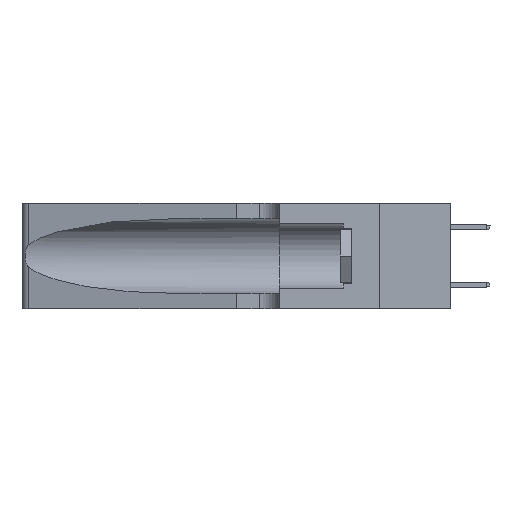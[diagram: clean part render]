
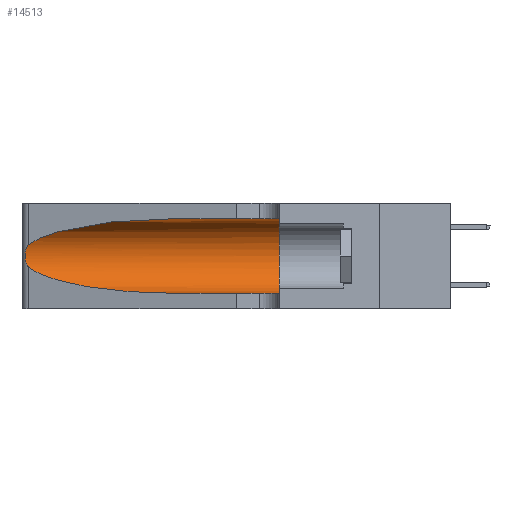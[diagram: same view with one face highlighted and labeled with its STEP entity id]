
A CAD part, left-side view. The second image highlights one B-rep face of the part: STEP entity #14513.
In plain terms, the highlighted cylindrical face has radius 3.308 mm (diameter 6.617 mm), a partial arc.
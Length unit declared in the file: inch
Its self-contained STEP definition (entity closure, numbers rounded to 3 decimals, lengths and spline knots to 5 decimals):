
#110 = DIRECTION ( 'NONE',  ( 0., -1., 0. ) ) ;
#166 = CIRCLE ( 'NONE', #18232, 0.13025 ) ;
#300 = LINE ( 'NONE', #17648, #17680 ) ;
#466 = EDGE_CURVE ( 'NONE', #22227, #18859, #23369, .T. ) ;
#804 = CARTESIAN_POINT ( 'NONE',  ( 0.25639, 1.23184, 0.21858 ) ) ;
#888 = ORIENTED_EDGE ( 'NONE', *, *, #16336, .F. ) ;
#924 = DIRECTION ( 'NONE',  ( 0., 0., -1. ) ) ;
#2369 = ORIENTED_EDGE ( 'NONE', *, *, #466, .T. ) ;
#2745 = VECTOR ( 'NONE', #110, 39.37008 ) ;
#2759 = VERTEX_POINT ( 'NONE', #21472 ) ;
#2931 = CARTESIAN_POINT ( 'NONE',  ( 0.26075, 1.23896, 0.178 ) ) ;
#5350 = VERTEX_POINT ( 'NONE', #18306 ) ;
#6581 = CARTESIAN_POINT ( 'NONE',  ( 0.25487, 1.22718, 0.14631 ) ) ;
#6843 = CYLINDRICAL_SURFACE ( 'NONE', #21247, 0.13025 ) ;
#7095 = CARTESIAN_POINT ( 'NONE',  ( 0.1305, 0.72297, 0.05475 ) ) ;
#8131 =( BOUNDED_CURVE ( )  B_SPLINE_CURVE ( 3, ( #22551, #12999, #22797, #11253 ),
 .UNSPECIFIED., .F., .F. ) 
 B_SPLINE_CURVE_WITH_KNOTS ( ( 4, 4 ),
 ( 1.5708, 2.84003 ),
 .UNSPECIFIED. ) 
 CURVE ( )  GEOMETRIC_REPRESENTATION_ITEM ( )  RATIONAL_B_SPLINE_CURVE ( ( 1., 0.87, 0.87, 1. ) ) 
 REPRESENTATION_ITEM ( '' )  );
#8192 = EDGE_LOOP ( 'NONE', ( #17746, #2369, #16391, #24027, #888, #19380 ) ) ;
#8236 = CARTESIAN_POINT ( 'NONE',  ( 0.25487, 1.22718, 0.22369 ) ) ;
#8818 = LINE ( 'NONE', #20715, #2745 ) ;
#8827 = CARTESIAN_POINT ( 'NONE',  ( 0.1305, 0.35, 0.185 ) ) ;
#10013 = CARTESIAN_POINT ( 'NONE',  ( 0.1305, 0.72297, 0.05475 ) ) ;
#10617 = CARTESIAN_POINT ( 'NONE',  ( 0.25487, 1.22718, 0.14631 ) ) ;
#10683 =( BOUNDED_CURVE ( )  B_SPLINE_CURVE ( 3, ( #10617, #10859, #10736, #7095 ),
 .UNSPECIFIED., .F., .T. ) 
 B_SPLINE_CURVE_WITH_KNOTS ( ( 4, 4 ),
 ( 3.44316, 4.71239 ),
 .UNSPECIFIED. ) 
 CURVE ( )  GEOMETRIC_REPRESENTATION_ITEM ( )  RATIONAL_B_SPLINE_CURVE ( ( 1., 0.87, 0.87, 1. ) ) 
 REPRESENTATION_ITEM ( '' )  );
#10736 = CARTESIAN_POINT ( 'NONE',  ( 0.18966, 0.96281, 0.05475 ) ) ;
#10859 = CARTESIAN_POINT ( 'NONE',  ( 0.2373, 1.15595, 0.08982 ) ) ;
#11253 = CARTESIAN_POINT ( 'NONE',  ( 0.25487, 1.22718, 0.22369 ) ) ;
#11676 = CARTESIAN_POINT ( 'NONE',  ( 0.25487, 1.22718, 0.14631 ) ) ;
#12350 = CARTESIAN_POINT ( 'NONE',  ( 0.1305, 0.72297, 0.31525 ) ) ;
#12591 = DIRECTION ( 'NONE',  ( 0., -1., 0. ) ) ;
#12599 = VERTEX_POINT ( 'NONE', #10013 ) ;
#12999 = CARTESIAN_POINT ( 'NONE',  ( 0.18966, 0.96281, 0.31525 ) ) ;
#13373 = EDGE_CURVE ( 'NONE', #12599, #2759, #8818, .T. ) ;
#13858 = CARTESIAN_POINT ( 'NONE',  ( 0.25787, 1.23484, 0.2124 ) ) ;
#14202 = DIRECTION ( 'NONE',  ( 0., 0., 1. ) ) ;
#14463 = CARTESIAN_POINT ( 'NONE',  ( 0.25487, 1.22718, 0.22369 ) ) ;
#14513 = ADVANCED_FACE ( 'NONE', ( #21786 ), #6843, .F. ) ;
#15771 = EDGE_CURVE ( 'NONE', #18040, #5350, #300, .T. ) ;
#15882 = CARTESIAN_POINT ( 'NONE',  ( 0.26017, 1.23833, 0.17102 ) ) ;
#16336 = EDGE_CURVE ( 'NONE', #5350, #2759, #166, .T. ) ;
#16391 = ORIENTED_EDGE ( 'NONE', *, *, #23026, .T. ) ;
#17648 = CARTESIAN_POINT ( 'NONE',  ( 0.1305, 1.61858, 0.31525 ) ) ;
#17680 = VECTOR ( 'NONE', #21291, 39.37008 ) ;
#17746 = ORIENTED_EDGE ( 'NONE', *, *, #22714, .T. ) ;
#18040 = VERTEX_POINT ( 'NONE', #12350 ) ;
#18232 = AXIS2_PLACEMENT_3D ( 'NONE', #8827, #23772, #14202 ) ;
#18265 = CARTESIAN_POINT ( 'NONE',  ( 0.1305, 1.61858, 0.185 ) ) ;
#18306 = CARTESIAN_POINT ( 'NONE',  ( 0.1305, 0.35, 0.31525 ) ) ;
#18859 = VERTEX_POINT ( 'NONE', #11676 ) ;
#19380 = ORIENTED_EDGE ( 'NONE', *, *, #15771, .F. ) ;
#19653 = CARTESIAN_POINT ( 'NONE',  ( 0.25555, 1.22994, 0.2215 ) ) ;
#20027 = CARTESIAN_POINT ( 'NONE',  ( 0.25555, 1.22993, 0.14849 ) ) ;
#20715 = CARTESIAN_POINT ( 'NONE',  ( 0.1305, 1.61858, 0.05475 ) ) ;
#21247 = AXIS2_PLACEMENT_3D ( 'NONE', #18265, #12591, #924 ) ;
#21291 = DIRECTION ( 'NONE',  ( 0., -1., 0. ) ) ;
#21472 = CARTESIAN_POINT ( 'NONE',  ( 0.1305, 0.35, 0.05475 ) ) ;
#21528 = CARTESIAN_POINT ( 'NONE',  ( 0.25789, 1.23486, 0.15765 ) ) ;
#21666 = CARTESIAN_POINT ( 'NONE',  ( 0.25856, 1.23593, 0.16098 ) ) ;
#21786 = FACE_OUTER_BOUND ( 'NONE', #8192, .T. ) ;
#21904 = CARTESIAN_POINT ( 'NONE',  ( 0.26018, 1.23835, 0.19895 ) ) ;
#22227 = VERTEX_POINT ( 'NONE', #14463 ) ;
#22551 = CARTESIAN_POINT ( 'NONE',  ( 0.1305, 0.72297, 0.31525 ) ) ;
#22714 = EDGE_CURVE ( 'NONE', #18040, #22227, #8131, .T. ) ;
#22797 = CARTESIAN_POINT ( 'NONE',  ( 0.2373, 1.15595, 0.28018 ) ) ;
#23026 = EDGE_CURVE ( 'NONE', #18859, #12599, #10683, .T. ) ;
#23369 = B_SPLINE_CURVE_WITH_KNOTS ( 'NONE', 3,
 ( #8236, #19653, #804, #13858, #23676, #21904, #23793, #2931, #15882, #21666, #21528, #23542, #20027, #6581 ),
 .UNSPECIFIED., .F., .F.,
 ( 4, 2, 2, 2, 2, 2, 4 ),
 ( 0., 0.00027, 0.00053, 0.00107, 0.0016, 0.00187, 0.00214 ),
 .UNSPECIFIED. ) ;
#23542 = CARTESIAN_POINT ( 'NONE',  ( 0.25639, 1.23186, 0.15144 ) ) ;
#23676 = CARTESIAN_POINT ( 'NONE',  ( 0.25854, 1.2359, 0.20912 ) ) ;
#23772 = DIRECTION ( 'NONE',  ( 0., 1., 0. ) ) ;
#23793 = CARTESIAN_POINT ( 'NONE',  ( 0.26075, 1.23896, 0.19203 ) ) ;
#24027 = ORIENTED_EDGE ( 'NONE', *, *, #13373, .T. ) ;
